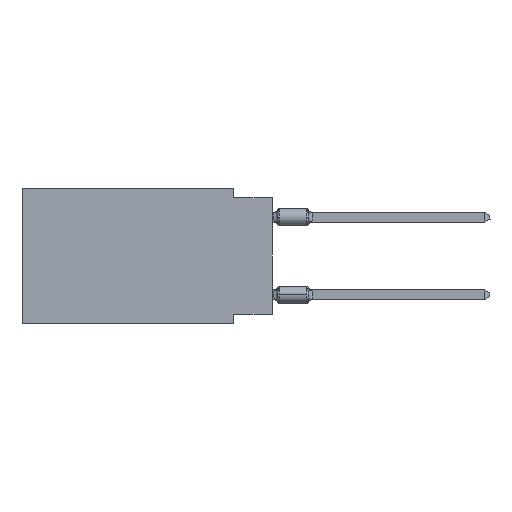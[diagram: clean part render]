
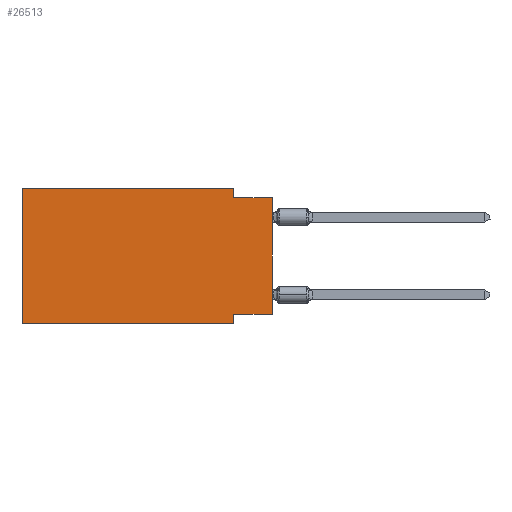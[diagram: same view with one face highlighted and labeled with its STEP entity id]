
A CAD part, left-side view. The second image highlights one B-rep face of the part: STEP entity #26513.
In plain terms, the highlighted planar face has unit normal (-1, 0, 0).
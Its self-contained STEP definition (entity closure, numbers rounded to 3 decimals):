
#1771 = FACE_OUTER_BOUND ( 'NONE', #8900, .T. ) ;
#2600 = ORIENTED_EDGE ( 'NONE', *, *, #3383, .F. ) ;
#2869 = CARTESIAN_POINT ( 'NONE',  ( 0., 16.383, 0. ) ) ;
#2902 = EDGE_CURVE ( 'NONE', #39578, #30636, #35417, .T. ) ;
#3383 = EDGE_CURVE ( 'NONE', #29827, #22354, #26301, .T. ) ;
#3762 = EDGE_CURVE ( 'NONE', #37688, #39578, #37733, .T. ) ;
#4270 = VECTOR ( 'NONE', #28691, 1000. ) ;
#4526 = LINE ( 'NONE', #19234, #4270 ) ;
#4663 = ORIENTED_EDGE ( 'NONE', *, *, #2902, .F. ) ;
#5545 = DIRECTION ( 'NONE',  ( 0., -1., 0. ) ) ;
#7411 = DIRECTION ( 'NONE',  ( 0., 0., -1. ) ) ;
#7448 = VERTEX_POINT ( 'NONE', #22447 ) ;
#8346 = ORIENTED_EDGE ( 'NONE', *, *, #3762, .F. ) ;
#8582 = EDGE_CURVE ( 'NONE', #33885, #29827, #4526, .T. ) ;
#8900 = EDGE_LOOP ( 'NONE', ( #30066, #38334, #2600, #21411, #39765, #30471, #4663, #8346 ) ) ;
#9655 = VECTOR ( 'NONE', #11024, 1000. ) ;
#10129 = CARTESIAN_POINT ( 'NONE',  ( 0., 2.54, -8.89 ) ) ;
#10839 = CARTESIAN_POINT ( 'NONE',  ( 0., 16.383, 0. ) ) ;
#11024 = DIRECTION ( 'NONE',  ( 0., 0., -1. ) ) ;
#11792 = LINE ( 'NONE', #35543, #37239 ) ;
#11885 = CARTESIAN_POINT ( 'NONE',  ( 0., 16.383, -8.89 ) ) ;
#15138 = DIRECTION ( 'NONE',  ( 0., 0., 1. ) ) ;
#15169 = EDGE_CURVE ( 'NONE', #38532, #30636, #11792, .T. ) ;
#15569 = CARTESIAN_POINT ( 'NONE',  ( 0., 0., -0.635 ) ) ;
#18626 = VECTOR ( 'NONE', #31074, 1000. ) ;
#18984 = CARTESIAN_POINT ( 'NONE',  ( 0., 0., 0. ) ) ;
#19234 = CARTESIAN_POINT ( 'NONE',  ( 0., 16.383, 0. ) ) ;
#19548 = CARTESIAN_POINT ( 'NONE',  ( 0., 2.54, -8.255 ) ) ;
#19610 = CARTESIAN_POINT ( 'NONE',  ( 0., 0., -8.255 ) ) ;
#20920 = VECTOR ( 'NONE', #15138, 1000. ) ;
#21216 = DIRECTION ( 'NONE',  ( 0., -1., 0. ) ) ;
#21335 = CARTESIAN_POINT ( 'NONE',  ( 0., 2.54, -0.635 ) ) ;
#21411 = ORIENTED_EDGE ( 'NONE', *, *, #8582, .F. ) ;
#22354 = VERTEX_POINT ( 'NONE', #21335 ) ;
#22447 = CARTESIAN_POINT ( 'NONE',  ( 0., 0., -0.635 ) ) ;
#22927 = CARTESIAN_POINT ( 'NONE',  ( 0., 2.54, -8.89 ) ) ;
#23051 = EDGE_CURVE ( 'NONE', #38532, #33885, #39304, .T. ) ;
#23494 = CARTESIAN_POINT ( 'NONE',  ( 0., 2.54, 0. ) ) ;
#26301 = LINE ( 'NONE', #38581, #9655 ) ;
#26353 = DIRECTION ( 'NONE',  ( 0., 0., -1. ) ) ;
#26513 = ADVANCED_FACE ( 'NONE', ( #1771 ), #34982, .F. ) ;
#27168 = EDGE_CURVE ( 'NONE', #37688, #7448, #37511, .T. ) ;
#28691 = DIRECTION ( 'NONE',  ( 0., -1., 0. ) ) ;
#29827 = VERTEX_POINT ( 'NONE', #23494 ) ;
#30066 = ORIENTED_EDGE ( 'NONE', *, *, #27168, .T. ) ;
#30471 = ORIENTED_EDGE ( 'NONE', *, *, #15169, .T. ) ;
#30636 = VERTEX_POINT ( 'NONE', #10129 ) ;
#31074 = DIRECTION ( 'NONE',  ( 0., 0., 1. ) ) ;
#31855 = EDGE_CURVE ( 'NONE', #22354, #7448, #39523, .T. ) ;
#32080 = AXIS2_PLACEMENT_3D ( 'NONE', #10839, #32757, #7411 ) ;
#32097 = VECTOR ( 'NONE', #26353, 1000. ) ;
#32757 = DIRECTION ( 'NONE',  ( 1., 0., 0. ) ) ;
#33885 = VERTEX_POINT ( 'NONE', #36324 ) ;
#34982 = PLANE ( 'NONE',  #32080 ) ;
#35109 = DIRECTION ( 'NONE',  ( 0., 1., 0. ) ) ;
#35417 = LINE ( 'NONE', #22927, #32097 ) ;
#35543 = CARTESIAN_POINT ( 'NONE',  ( 0., 16.383, -8.89 ) ) ;
#36324 = CARTESIAN_POINT ( 'NONE',  ( 0., 16.383, 0. ) ) ;
#37239 = VECTOR ( 'NONE', #5545, 1000. ) ;
#37332 = VECTOR ( 'NONE', #35109, 1000. ) ;
#37511 = LINE ( 'NONE', #18984, #18626 ) ;
#37688 = VERTEX_POINT ( 'NONE', #39147 ) ;
#37733 = LINE ( 'NONE', #19610, #37332 ) ;
#38334 = ORIENTED_EDGE ( 'NONE', *, *, #31855, .F. ) ;
#38532 = VERTEX_POINT ( 'NONE', #11885 ) ;
#38581 = CARTESIAN_POINT ( 'NONE',  ( 0., 2.54, 0. ) ) ;
#39147 = CARTESIAN_POINT ( 'NONE',  ( 0., 0., -8.255 ) ) ;
#39304 = LINE ( 'NONE', #2869, #20920 ) ;
#39523 = LINE ( 'NONE', #15569, #39733 ) ;
#39578 = VERTEX_POINT ( 'NONE', #19548 ) ;
#39733 = VECTOR ( 'NONE', #21216, 1000. ) ;
#39765 = ORIENTED_EDGE ( 'NONE', *, *, #23051, .F. ) ;
